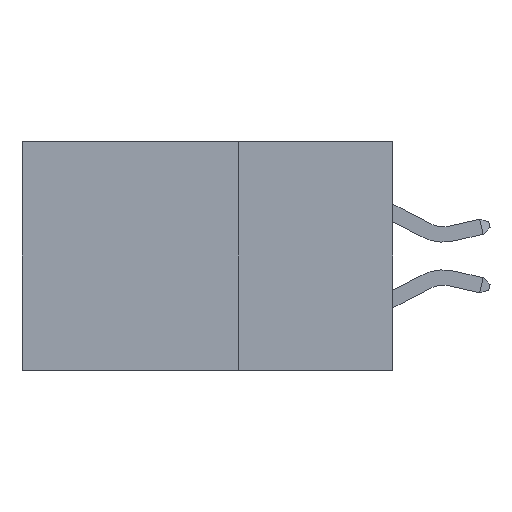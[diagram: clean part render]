
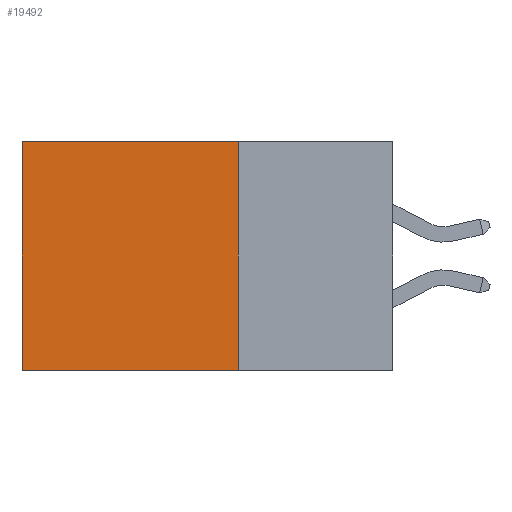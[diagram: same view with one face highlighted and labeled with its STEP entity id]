
A CAD part, left-side view. The second image highlights one B-rep face of the part: STEP entity #19492.
In plain terms, the highlighted planar face has unit normal (-1, 0, 0).
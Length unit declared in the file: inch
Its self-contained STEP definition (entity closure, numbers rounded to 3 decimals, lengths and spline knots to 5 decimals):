
#791 = CARTESIAN_POINT ( 'NONE',  ( 0.2875, 0.25, -0.37 ) ) ;
#1471 = CARTESIAN_POINT ( 'NONE',  ( 0.2875, 0.25, 0. ) ) ;
#3288 = AXIS2_PLACEMENT_3D ( 'NONE', #17146, #29004, #31937 ) ;
#4401 = DIRECTION ( 'NONE',  ( 0., 0., -1. ) ) ;
#5346 = ORIENTED_EDGE ( 'NONE', *, *, #18019, .T. ) ;
#6514 = VECTOR ( 'NONE', #4401, 39.37008 ) ;
#7110 = CARTESIAN_POINT ( 'NONE',  ( 0.2875, 0.6, 0. ) ) ;
#8339 = VECTOR ( 'NONE', #24980, 39.37008 ) ;
#11213 = VECTOR ( 'NONE', #30877, 39.37008 ) ;
#12596 = LINE ( 'NONE', #13539, #20337 ) ;
#13539 = CARTESIAN_POINT ( 'NONE',  ( 0.2875, 0.25, -0.37 ) ) ;
#14441 = VERTEX_POINT ( 'NONE', #16005 ) ;
#16005 = CARTESIAN_POINT ( 'NONE',  ( 0.2875, 0.25, 0. ) ) ;
#17146 = CARTESIAN_POINT ( 'NONE',  ( 0.2875, 0.25, 0. ) ) ;
#18019 = EDGE_CURVE ( 'NONE', #14441, #26758, #26158, .T. ) ;
#18793 = LINE ( 'NONE', #7110, #6514 ) ;
#19247 = EDGE_CURVE ( 'NONE', #26758, #31111, #18793, .T. ) ;
#19492 = ADVANCED_FACE ( 'NONE', ( #21064 ), #31802, .F. ) ;
#19864 = LINE ( 'NONE', #22080, #11213 ) ;
#20337 = VECTOR ( 'NONE', #30865, 39.37008 ) ;
#21064 = FACE_OUTER_BOUND ( 'NONE', #34896, .T. ) ;
#21512 = ORIENTED_EDGE ( 'NONE', *, *, #26956, .F. ) ;
#22080 = CARTESIAN_POINT ( 'NONE',  ( 0.2875, 0.25, 0. ) ) ;
#22544 = EDGE_CURVE ( 'NONE', #14441, #35791, #19864, .T. ) ;
#24641 = ORIENTED_EDGE ( 'NONE', *, *, #19247, .T. ) ;
#24980 = DIRECTION ( 'NONE',  ( 0., 1., 0. ) ) ;
#26158 = LINE ( 'NONE', #1471, #8339 ) ;
#26479 = CARTESIAN_POINT ( 'NONE',  ( 0.2875, 0.6, 0. ) ) ;
#26758 = VERTEX_POINT ( 'NONE', #26479 ) ;
#26956 = EDGE_CURVE ( 'NONE', #35791, #31111, #12596, .T. ) ;
#29004 = DIRECTION ( 'NONE',  ( 1., 0., 0. ) ) ;
#29138 = CARTESIAN_POINT ( 'NONE',  ( 0.2875, 0.6, -0.37 ) ) ;
#30865 = DIRECTION ( 'NONE',  ( 0., 1., 0. ) ) ;
#30877 = DIRECTION ( 'NONE',  ( 0., 0., -1. ) ) ;
#31111 = VERTEX_POINT ( 'NONE', #29138 ) ;
#31802 = PLANE ( 'NONE',  #3288 ) ;
#31937 = DIRECTION ( 'NONE',  ( 0., 0., -1. ) ) ;
#34896 = EDGE_LOOP ( 'NONE', ( #24641, #21512, #36359, #5346 ) ) ;
#35791 = VERTEX_POINT ( 'NONE', #791 ) ;
#36359 = ORIENTED_EDGE ( 'NONE', *, *, #22544, .F. ) ;
